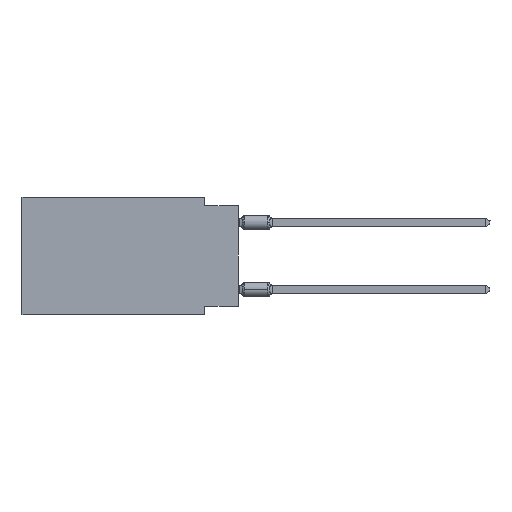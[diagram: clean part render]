
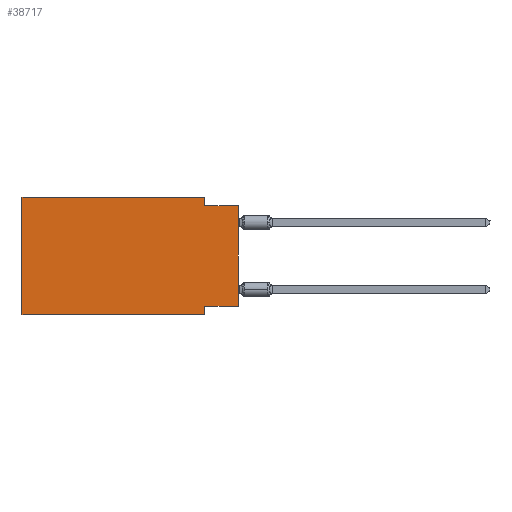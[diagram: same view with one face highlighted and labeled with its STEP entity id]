
A CAD part, left-side view. The second image highlights one B-rep face of the part: STEP entity #38717.
In plain terms, the highlighted planar face has unit normal (-1, 0, 0).
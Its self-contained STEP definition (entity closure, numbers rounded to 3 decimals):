
#1351 = DIRECTION ( 'NONE',  ( 0., -1., 0. ) ) ;
#1936 = CARTESIAN_POINT ( 'NONE',  ( 0., 0., -8.255 ) ) ;
#2129 = EDGE_CURVE ( 'NONE', #57923, #16455, #16534, .T. ) ;
#2578 = CARTESIAN_POINT ( 'NONE',  ( 0., 2.54, -8.89 ) ) ;
#2882 = VECTOR ( 'NONE', #70766, 1000. ) ;
#6002 = FACE_OUTER_BOUND ( 'NONE', #63261, .T. ) ;
#6471 = LINE ( 'NONE', #48543, #2882 ) ;
#8965 = CARTESIAN_POINT ( 'NONE',  ( 0., 16.383, 0. ) ) ;
#10817 = DIRECTION ( 'NONE',  ( 0., -1., 0. ) ) ;
#12255 = ORIENTED_EDGE ( 'NONE', *, *, #24590, .F. ) ;
#13010 = CARTESIAN_POINT ( 'NONE',  ( 0., 16.383, 0. ) ) ;
#13137 = VERTEX_POINT ( 'NONE', #16447 ) ;
#13444 = CARTESIAN_POINT ( 'NONE',  ( 0., 2.54, 0. ) ) ;
#13460 = EDGE_CURVE ( 'NONE', #67020, #55138, #51311, .T. ) ;
#14878 = LINE ( 'NONE', #37117, #71812 ) ;
#16447 = CARTESIAN_POINT ( 'NONE',  ( 0., 2.54, -8.255 ) ) ;
#16455 = VERTEX_POINT ( 'NONE', #48980 ) ;
#16534 = LINE ( 'NONE', #70512, #43622 ) ;
#17821 = LINE ( 'NONE', #67390, #65054 ) ;
#20261 = LINE ( 'NONE', #8965, #37216 ) ;
#21077 = CARTESIAN_POINT ( 'NONE',  ( 0., 0., -0.635 ) ) ;
#22016 = CARTESIAN_POINT ( 'NONE',  ( 0., 16.383, 0. ) ) ;
#22691 = ORIENTED_EDGE ( 'NONE', *, *, #45408, .F. ) ;
#24590 = EDGE_CURVE ( 'NONE', #55138, #71595, #6471, .T. ) ;
#27894 = DIRECTION ( 'NONE',  ( 1., 0., 0. ) ) ;
#28244 = CARTESIAN_POINT ( 'NONE',  ( 0., 16.383, 0. ) ) ;
#28669 = ORIENTED_EDGE ( 'NONE', *, *, #51201, .T. ) ;
#28901 = AXIS2_PLACEMENT_3D ( 'NONE', #28244, #27894, #34064 ) ;
#29465 = VERTEX_POINT ( 'NONE', #46014 ) ;
#30363 = CARTESIAN_POINT ( 'NONE',  ( 0., 16.383, -8.89 ) ) ;
#31202 = DIRECTION ( 'NONE',  ( 0., 0., 1. ) ) ;
#31510 = DIRECTION ( 'NONE',  ( 0., -1., 0. ) ) ;
#31885 = EDGE_CURVE ( 'NONE', #13137, #16455, #57653, .T. ) ;
#33791 = EDGE_CURVE ( 'NONE', #71595, #29465, #66236, .T. ) ;
#33899 = VECTOR ( 'NONE', #68228, 1000. ) ;
#34064 = DIRECTION ( 'NONE',  ( 0., 0., -1. ) ) ;
#34088 = VECTOR ( 'NONE', #10817, 1000. ) ;
#37117 = CARTESIAN_POINT ( 'NONE',  ( 0., 0., 0. ) ) ;
#37216 = VECTOR ( 'NONE', #31202, 1000. ) ;
#38717 = ADVANCED_FACE ( 'NONE', ( #6002 ), #44660, .F. ) ;
#39297 = EDGE_CURVE ( 'NONE', #58014, #13137, #17821, .T. ) ;
#43622 = VECTOR ( 'NONE', #31510, 1000. ) ;
#44660 = PLANE ( 'NONE',  #28901 ) ;
#45408 = EDGE_CURVE ( 'NONE', #57923, #67020, #20261, .T. ) ;
#46014 = CARTESIAN_POINT ( 'NONE',  ( 0., 0., -0.635 ) ) ;
#48543 = CARTESIAN_POINT ( 'NONE',  ( 0., 2.54, 0. ) ) ;
#48980 = CARTESIAN_POINT ( 'NONE',  ( 0., 2.54, -8.89 ) ) ;
#51201 = EDGE_CURVE ( 'NONE', #58014, #29465, #14878, .T. ) ;
#51311 = LINE ( 'NONE', #13010, #62016 ) ;
#55032 = ORIENTED_EDGE ( 'NONE', *, *, #39297, .F. ) ;
#55138 = VERTEX_POINT ( 'NONE', #13444 ) ;
#55586 = ORIENTED_EDGE ( 'NONE', *, *, #2129, .T. ) ;
#57653 = LINE ( 'NONE', #2578, #33899 ) ;
#57723 = ORIENTED_EDGE ( 'NONE', *, *, #31885, .F. ) ;
#57923 = VERTEX_POINT ( 'NONE', #30363 ) ;
#58014 = VERTEX_POINT ( 'NONE', #1936 ) ;
#59360 = DIRECTION ( 'NONE',  ( 0., 0., 1. ) ) ;
#60261 = ORIENTED_EDGE ( 'NONE', *, *, #33791, .F. ) ;
#62016 = VECTOR ( 'NONE', #1351, 1000. ) ;
#63010 = DIRECTION ( 'NONE',  ( 0., 1., 0. ) ) ;
#63261 = EDGE_LOOP ( 'NONE', ( #28669, #60261, #12255, #63634, #22691, #55586, #57723, #55032 ) ) ;
#63634 = ORIENTED_EDGE ( 'NONE', *, *, #13460, .F. ) ;
#65054 = VECTOR ( 'NONE', #63010, 1000. ) ;
#66236 = LINE ( 'NONE', #21077, #34088 ) ;
#67020 = VERTEX_POINT ( 'NONE', #22016 ) ;
#67047 = CARTESIAN_POINT ( 'NONE',  ( 0., 2.54, -0.635 ) ) ;
#67390 = CARTESIAN_POINT ( 'NONE',  ( 0., 0., -8.255 ) ) ;
#68228 = DIRECTION ( 'NONE',  ( 0., 0., -1. ) ) ;
#70512 = CARTESIAN_POINT ( 'NONE',  ( 0., 16.383, -8.89 ) ) ;
#70766 = DIRECTION ( 'NONE',  ( 0., 0., -1. ) ) ;
#71595 = VERTEX_POINT ( 'NONE', #67047 ) ;
#71812 = VECTOR ( 'NONE', #59360, 1000. ) ;
